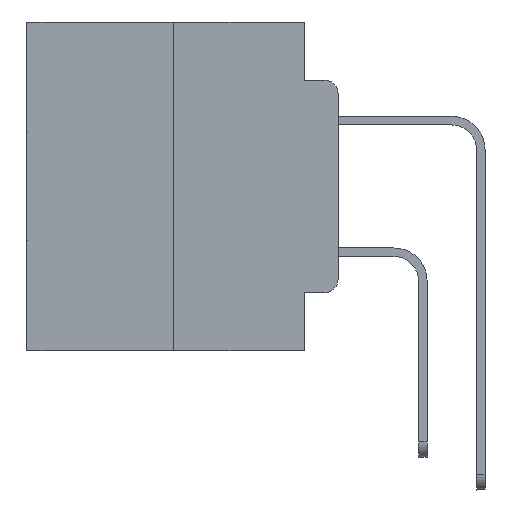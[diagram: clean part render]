
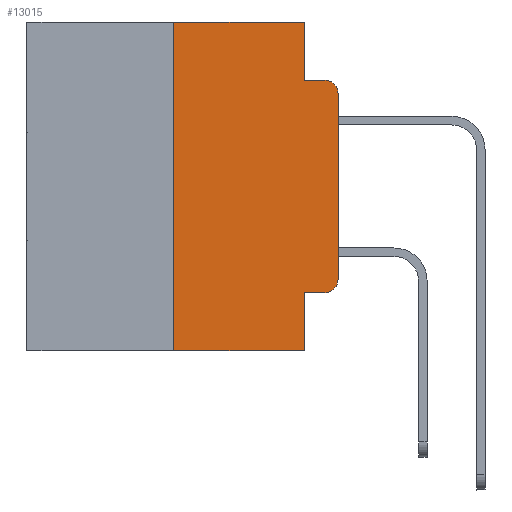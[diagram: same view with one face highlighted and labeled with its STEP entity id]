
A CAD part, left-side view. The second image highlights one B-rep face of the part: STEP entity #13015.
In plain terms, the highlighted planar face has unit normal (-1, 0, 0).
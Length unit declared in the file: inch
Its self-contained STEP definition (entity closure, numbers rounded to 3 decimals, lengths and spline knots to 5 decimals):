
#525 = VERTEX_POINT ( 'NONE', #7823 ) ;
#1123 = VERTEX_POINT ( 'NONE', #23898 ) ;
#1570 = DIRECTION ( 'NONE',  ( 0., 0., -1. ) ) ;
#2074 = VECTOR ( 'NONE', #1570, 39.37008 ) ;
#2314 = CARTESIAN_POINT ( 'NONE',  ( 0., 0.051, -0.4115 ) ) ;
#2371 = ORIENTED_EDGE ( 'NONE', *, *, #11820, .T. ) ;
#3214 = DIRECTION ( 'NONE',  ( 0., -1., 0. ) ) ;
#3946 = CARTESIAN_POINT ( 'NONE',  ( 0., 0.051, 0. ) ) ;
#4080 = DIRECTION ( 'NONE',  ( 0., -1., 0. ) ) ;
#4354 = LINE ( 'NONE', #8117, #22313 ) ;
#4772 = CIRCLE ( 'NONE', #6591, 0.02 ) ;
#4806 = CARTESIAN_POINT ( 'NONE',  ( 0., 0.02, -0.0885 ) ) ;
#4890 = CARTESIAN_POINT ( 'NONE',  ( 0., 0.02, -0.1085 ) ) ;
#5023 = PLANE ( 'NONE',  #21545 ) ;
#6050 = VECTOR ( 'NONE', #27218, 39.37008 ) ;
#6332 = CARTESIAN_POINT ( 'NONE',  ( 0., 0.051, 0. ) ) ;
#6591 = AXIS2_PLACEMENT_3D ( 'NONE', #25592, #12335, #27755 ) ;
#6657 = EDGE_CURVE ( 'NONE', #27944, #26971, #24272, .T. ) ;
#7222 = DIRECTION ( 'NONE',  ( 0., 0., -1. ) ) ;
#7263 = ORIENTED_EDGE ( 'NONE', *, *, #6657, .F. ) ;
#7413 = EDGE_CURVE ( 'NONE', #1123, #25581, #16366, .T. ) ;
#7735 = LINE ( 'NONE', #6332, #19697 ) ;
#7817 = ORIENTED_EDGE ( 'NONE', *, *, #25779, .F. ) ;
#7823 = CARTESIAN_POINT ( 'NONE',  ( 0., 0.25, 0. ) ) ;
#8117 = CARTESIAN_POINT ( 'NONE',  ( 0., 0.473, -0.5 ) ) ;
#9679 = AXIS2_PLACEMENT_3D ( 'NONE', #4890, #20672, #7222 ) ;
#9749 = DIRECTION ( 'NONE',  ( 1., 0., 0. ) ) ;
#10153 = LINE ( 'NONE', #14182, #16138 ) ;
#11820 = EDGE_CURVE ( 'NONE', #28294, #28523, #4354, .T. ) ;
#11999 = CARTESIAN_POINT ( 'NONE',  ( 0., 0.02, -0.4115 ) ) ;
#12108 = LINE ( 'NONE', #16302, #6050 ) ;
#12335 = DIRECTION ( 'NONE',  ( -1., 0., 0. ) ) ;
#13015 = ADVANCED_FACE ( 'NONE', ( #21632 ), #5023, .F. ) ;
#13965 = EDGE_CURVE ( 'NONE', #24152, #27944, #14270, .T. ) ;
#14179 = CARTESIAN_POINT ( 'NONE',  ( 0., 0.473, 0. ) ) ;
#14182 = CARTESIAN_POINT ( 'NONE',  ( 0., 0.473, 0. ) ) ;
#14270 = LINE ( 'NONE', #3946, #2074 ) ;
#14390 = CARTESIAN_POINT ( 'NONE',  ( 0., 0.051, -0.4115 ) ) ;
#16138 = VECTOR ( 'NONE', #16444, 39.37008 ) ;
#16302 = CARTESIAN_POINT ( 'NONE',  ( 0., 0.25, 0. ) ) ;
#16366 = LINE ( 'NONE', #22027, #27328 ) ;
#16444 = DIRECTION ( 'NONE',  ( 0., -1., 0. ) ) ;
#16650 = VERTEX_POINT ( 'NONE', #2314 ) ;
#16944 = CARTESIAN_POINT ( 'NONE',  ( 0., 0.25, -0.5 ) ) ;
#17914 = CARTESIAN_POINT ( 'NONE',  ( 0., 0.051, -0.0885 ) ) ;
#17955 = EDGE_CURVE ( 'NONE', #25581, #26971, #18419, .T. ) ;
#18369 = ORIENTED_EDGE ( 'NONE', *, *, #19938, .T. ) ;
#18419 = CIRCLE ( 'NONE', #9679, 0.02 ) ;
#19452 = ORIENTED_EDGE ( 'NONE', *, *, #28722, .F. ) ;
#19697 = VECTOR ( 'NONE', #19825, 39.37008 ) ;
#19825 = DIRECTION ( 'NONE',  ( 0., 0., -1. ) ) ;
#19938 = EDGE_CURVE ( 'NONE', #16650, #27520, #24186, .T. ) ;
#20672 = DIRECTION ( 'NONE',  ( -1., 0., 0. ) ) ;
#21154 = ORIENTED_EDGE ( 'NONE', *, *, #7413, .T. ) ;
#21252 = ORIENTED_EDGE ( 'NONE', *, *, #17955, .T. ) ;
#21545 = AXIS2_PLACEMENT_3D ( 'NONE', #14179, #9749, #25281 ) ;
#21632 = FACE_OUTER_BOUND ( 'NONE', #27003, .T. ) ;
#22027 = CARTESIAN_POINT ( 'NONE',  ( 0., 0., 0. ) ) ;
#22207 = DIRECTION ( 'NONE',  ( 0., 0., 1. ) ) ;
#22313 = VECTOR ( 'NONE', #23736, 39.37008 ) ;
#23406 = CARTESIAN_POINT ( 'NONE',  ( 0., 0.051, 0. ) ) ;
#23736 = DIRECTION ( 'NONE',  ( 0., -1., 0. ) ) ;
#23898 = CARTESIAN_POINT ( 'NONE',  ( 0., 0., -0.3915 ) ) ;
#24152 = VERTEX_POINT ( 'NONE', #23406 ) ;
#24186 = LINE ( 'NONE', #14390, #28593 ) ;
#24272 = LINE ( 'NONE', #27533, #24959 ) ;
#24424 = CARTESIAN_POINT ( 'NONE',  ( 0., 0.051, -0.5 ) ) ;
#24751 = ORIENTED_EDGE ( 'NONE', *, *, #28242, .T. ) ;
#24959 = VECTOR ( 'NONE', #4080, 39.37008 ) ;
#25281 = DIRECTION ( 'NONE',  ( 0., 0., -1. ) ) ;
#25581 = VERTEX_POINT ( 'NONE', #26552 ) ;
#25592 = CARTESIAN_POINT ( 'NONE',  ( 0., 0.02, -0.3915 ) ) ;
#25779 = EDGE_CURVE ( 'NONE', #28294, #525, #12108, .T. ) ;
#26349 = ORIENTED_EDGE ( 'NONE', *, *, #13965, .F. ) ;
#26552 = CARTESIAN_POINT ( 'NONE',  ( 0., 0., -0.1085 ) ) ;
#26589 = ORIENTED_EDGE ( 'NONE', *, *, #27238, .F. ) ;
#26971 = VERTEX_POINT ( 'NONE', #4806 ) ;
#27003 = EDGE_LOOP ( 'NONE', ( #21154, #21252, #7263, #26349, #19452, #7817, #2371, #26589, #18369, #24751 ) ) ;
#27218 = DIRECTION ( 'NONE',  ( 0., 0., 1. ) ) ;
#27238 = EDGE_CURVE ( 'NONE', #16650, #28523, #7735, .T. ) ;
#27328 = VECTOR ( 'NONE', #22207, 39.37008 ) ;
#27520 = VERTEX_POINT ( 'NONE', #11999 ) ;
#27533 = CARTESIAN_POINT ( 'NONE',  ( 0., 0.051, -0.0885 ) ) ;
#27755 = DIRECTION ( 'NONE',  ( 0., 0., -1. ) ) ;
#27944 = VERTEX_POINT ( 'NONE', #17914 ) ;
#28242 = EDGE_CURVE ( 'NONE', #27520, #1123, #4772, .T. ) ;
#28294 = VERTEX_POINT ( 'NONE', #16944 ) ;
#28523 = VERTEX_POINT ( 'NONE', #24424 ) ;
#28593 = VECTOR ( 'NONE', #3214, 39.37008 ) ;
#28722 = EDGE_CURVE ( 'NONE', #525, #24152, #10153, .T. ) ;
